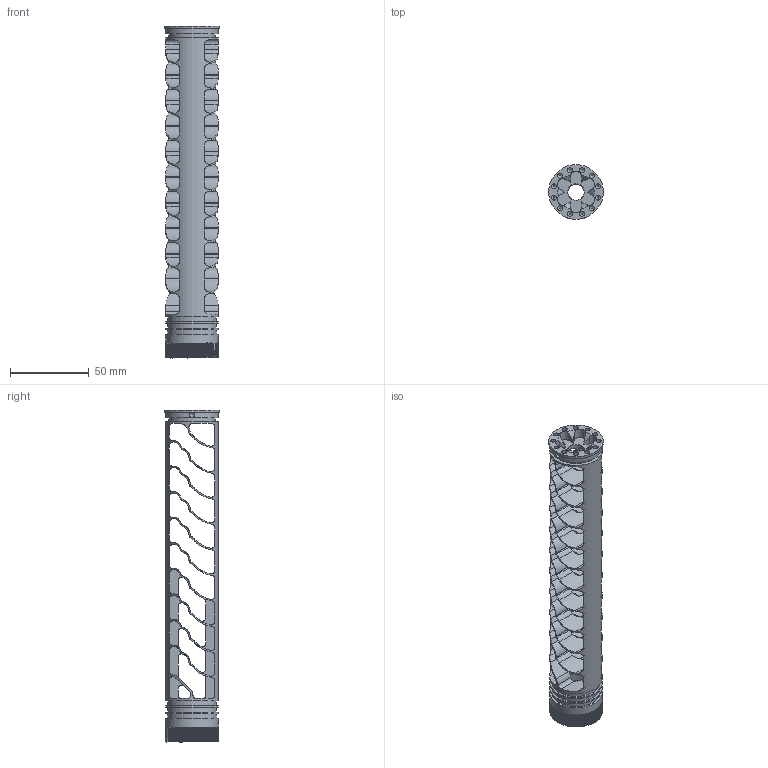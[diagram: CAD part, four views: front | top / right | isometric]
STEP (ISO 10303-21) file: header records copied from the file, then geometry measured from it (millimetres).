
FILE_DESCRIPTION (( 'STEP AP214' ), '1' );
FILE_NAME ('core.step', '2016-02-01T19:14:44', ( 'WarFairy' ), ( '' ), 'SwSTEP 2.0', 'SolidWorks 2015', '' );
FILE_SCHEMA (( 'AUTOMOTIVE_DESIGN' ));
Length unit declared in the file: inch
Products named in the file (1): core
Bounding box: 34.8 x 34.8 x 211.28 mm (x, y, z)
Volume: 27688.6 mm3; surface area: 46727.9 mm2
Topology: 1 solids, 1 shells, 434 faces, 1342 edges, 887 vertices
Faces by surface type: cylinder 294, plane 117, cone 19, bspline 4
Full cylindrical faces by diameter (mm): 3.175 x13, 10.5 x11, 28.905 x12, 29.337 x1, 30.861 x3, 33.401 x18, 34.798 x1
Entity records: 21279 total; most frequent: CARTESIAN_POINT 11372, ORIENTED_EDGE 2308, DIRECTION 1649, EDGE_CURVE 1154, VERTEX_POINT 785, AXIS2_PLACEMENT_3D 587, EDGE_LOOP 495, LINE 475
